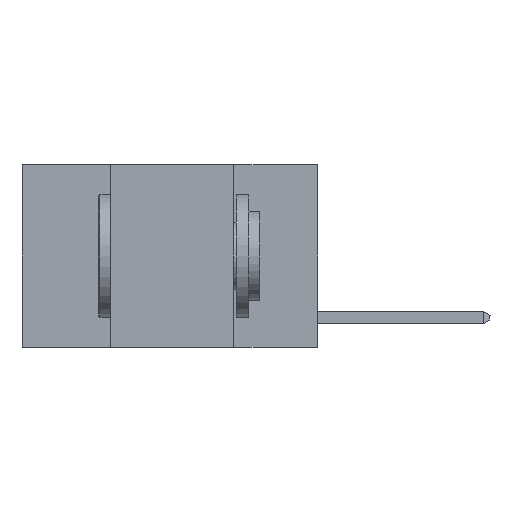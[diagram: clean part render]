
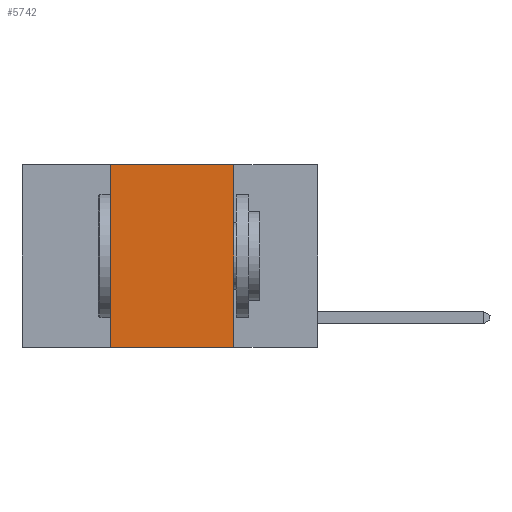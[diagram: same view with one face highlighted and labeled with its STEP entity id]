
A CAD part, left-side view. The second image highlights one B-rep face of the part: STEP entity #5742.
In plain terms, the highlighted planar face has unit normal (-1, 0, 0).
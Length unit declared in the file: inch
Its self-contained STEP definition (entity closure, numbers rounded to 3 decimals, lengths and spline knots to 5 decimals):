
#646 = EDGE_CURVE ( 'NONE', #2089, #3694, #9294, .T. ) ;
#867 = EDGE_CURVE ( 'NONE', #9659, #1705, #2309, .T. ) ;
#1114 = FACE_OUTER_BOUND ( 'NONE', #12844, .T. ) ;
#1299 = CARTESIAN_POINT ( 'NONE',  ( 0., 0.6, 0. ) ) ;
#1705 = VERTEX_POINT ( 'NONE', #17825 ) ;
#1743 = ORIENTED_EDGE ( 'NONE', *, *, #16701, .F. ) ;
#2089 = VERTEX_POINT ( 'NONE', #13733 ) ;
#2309 = LINE ( 'NONE', #15684, #10855 ) ;
#3694 = VERTEX_POINT ( 'NONE', #15811 ) ;
#4519 = LINE ( 'NONE', #7884, #13930 ) ;
#5220 = EDGE_CURVE ( 'NONE', #9659, #3694, #4519, .T. ) ;
#5650 = DIRECTION ( 'NONE',  ( 1., 0., 0. ) ) ;
#5716 = PLANE ( 'NONE',  #7747 ) ;
#5742 = ADVANCED_FACE ( 'NONE', ( #1114 ), #5716, .F. ) ;
#6268 = VECTOR ( 'NONE', #14584, 39.37008 ) ;
#7221 = DIRECTION ( 'NONE',  ( 0., 0., -1. ) ) ;
#7747 = AXIS2_PLACEMENT_3D ( 'NONE', #1299, #5650, #7221 ) ;
#7884 = CARTESIAN_POINT ( 'NONE',  ( 0., 0.6, -0.37 ) ) ;
#8453 = DIRECTION ( 'NONE',  ( 0., 0., 1. ) ) ;
#8958 = CARTESIAN_POINT ( 'NONE',  ( 0., 0.6, 0. ) ) ;
#9007 = ORIENTED_EDGE ( 'NONE', *, *, #867, .F. ) ;
#9294 = LINE ( 'NONE', #12988, #9768 ) ;
#9578 = CARTESIAN_POINT ( 'NONE',  ( 0., 0.42, -0.37 ) ) ;
#9659 = VERTEX_POINT ( 'NONE', #9578 ) ;
#9768 = VECTOR ( 'NONE', #10100, 39.37008 ) ;
#10077 = LINE ( 'NONE', #8958, #6268 ) ;
#10100 = DIRECTION ( 'NONE',  ( 0., 0., -1. ) ) ;
#10855 = VECTOR ( 'NONE', #8453, 39.37008 ) ;
#12147 = ORIENTED_EDGE ( 'NONE', *, *, #5220, .T. ) ;
#12844 = EDGE_LOOP ( 'NONE', ( #12961, #1743, #9007, #12147 ) ) ;
#12961 = ORIENTED_EDGE ( 'NONE', *, *, #646, .F. ) ;
#12988 = CARTESIAN_POINT ( 'NONE',  ( 0., 0.17, 0. ) ) ;
#13733 = CARTESIAN_POINT ( 'NONE',  ( 0., 0.17, 0. ) ) ;
#13930 = VECTOR ( 'NONE', #17954, 39.37008 ) ;
#14584 = DIRECTION ( 'NONE',  ( 0., -1., 0. ) ) ;
#15684 = CARTESIAN_POINT ( 'NONE',  ( 0., 0.42, 0. ) ) ;
#15811 = CARTESIAN_POINT ( 'NONE',  ( 0., 0.17, -0.37 ) ) ;
#16701 = EDGE_CURVE ( 'NONE', #1705, #2089, #10077, .T. ) ;
#17825 = CARTESIAN_POINT ( 'NONE',  ( 0., 0.42, 0. ) ) ;
#17954 = DIRECTION ( 'NONE',  ( 0., -1., 0. ) ) ;
